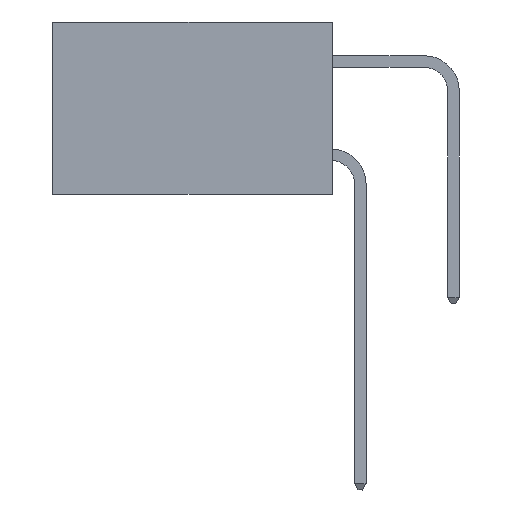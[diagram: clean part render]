
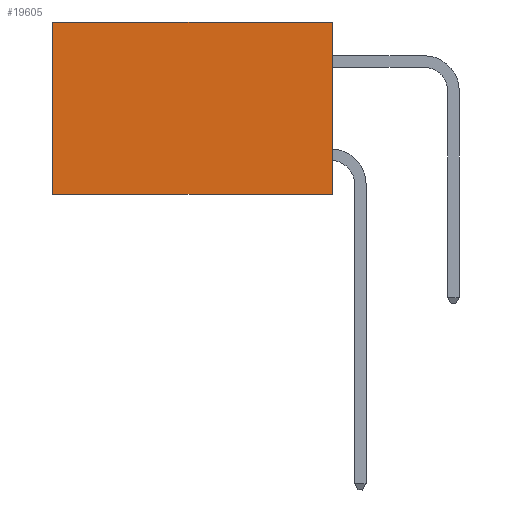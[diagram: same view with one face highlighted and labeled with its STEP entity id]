
A CAD part, left-side view. The second image highlights one B-rep face of the part: STEP entity #19605.
In plain terms, the highlighted planar face has unit normal (-1, 0, 0).
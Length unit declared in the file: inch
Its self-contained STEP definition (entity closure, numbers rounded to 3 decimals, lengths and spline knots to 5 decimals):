
#2109 = DIRECTION ( 'NONE',  ( 0., 0., -1. ) ) ;
#2380 = LINE ( 'NONE', #11107, #15554 ) ;
#2677 = ORIENTED_EDGE ( 'NONE', *, *, #19838, .T. ) ;
#3389 = ORIENTED_EDGE ( 'NONE', *, *, #23958, .F. ) ;
#4301 = VERTEX_POINT ( 'NONE', #8975 ) ;
#4640 = VERTEX_POINT ( 'NONE', #16150 ) ;
#5847 = FACE_OUTER_BOUND ( 'NONE', #22194, .T. ) ;
#6780 = CARTESIAN_POINT ( 'NONE',  ( 0.298, 0., 0. ) ) ;
#7789 = VECTOR ( 'NONE', #2109, 39.37008 ) ;
#8274 = ORIENTED_EDGE ( 'NONE', *, *, #14228, .T. ) ;
#8285 = CARTESIAN_POINT ( 'NONE',  ( 0.298, 0.6, 0. ) ) ;
#8975 = CARTESIAN_POINT ( 'NONE',  ( 0.298, 0., 0. ) ) ;
#9934 = VERTEX_POINT ( 'NONE', #27888 ) ;
#10993 = DIRECTION ( 'NONE',  ( 1., 0., 0. ) ) ;
#11107 = CARTESIAN_POINT ( 'NONE',  ( 0.298, 0., -0.37 ) ) ;
#13133 = LINE ( 'NONE', #6780, #7789 ) ;
#13181 = CARTESIAN_POINT ( 'NONE',  ( 0.298, 0., 0. ) ) ;
#13428 = ORIENTED_EDGE ( 'NONE', *, *, #29574, .F. ) ;
#14228 = EDGE_CURVE ( 'NONE', #4301, #9934, #21830, .T. ) ;
#15554 = VECTOR ( 'NONE', #15592, 39.37008 ) ;
#15592 = DIRECTION ( 'NONE',  ( 0., 1., 0. ) ) ;
#15764 = DIRECTION ( 'NONE',  ( 0., 0., -1. ) ) ;
#16150 = CARTESIAN_POINT ( 'NONE',  ( 0.298, 0.6, -0.37 ) ) ;
#16781 = AXIS2_PLACEMENT_3D ( 'NONE', #13181, #10993, #15764 ) ;
#17481 = DIRECTION ( 'NONE',  ( 0., 1., 0. ) ) ;
#19605 = ADVANCED_FACE ( 'NONE', ( #5847 ), #26853, .F. ) ;
#19838 = EDGE_CURVE ( 'NONE', #9934, #4640, #22296, .T. ) ;
#20006 = VERTEX_POINT ( 'NONE', #21421 ) ;
#20099 = VECTOR ( 'NONE', #26416, 39.37008 ) ;
#21421 = CARTESIAN_POINT ( 'NONE',  ( 0.298, 0., -0.37 ) ) ;
#21830 = LINE ( 'NONE', #28670, #27175 ) ;
#22194 = EDGE_LOOP ( 'NONE', ( #2677, #3389, #13428, #8274 ) ) ;
#22296 = LINE ( 'NONE', #8285, #20099 ) ;
#23958 = EDGE_CURVE ( 'NONE', #20006, #4640, #2380, .T. ) ;
#26416 = DIRECTION ( 'NONE',  ( 0., 0., -1. ) ) ;
#26853 = PLANE ( 'NONE',  #16781 ) ;
#27175 = VECTOR ( 'NONE', #17481, 39.37008 ) ;
#27888 = CARTESIAN_POINT ( 'NONE',  ( 0.298, 0.6, 0. ) ) ;
#28670 = CARTESIAN_POINT ( 'NONE',  ( 0.298, 0., 0. ) ) ;
#29574 = EDGE_CURVE ( 'NONE', #4301, #20006, #13133, .T. ) ;
